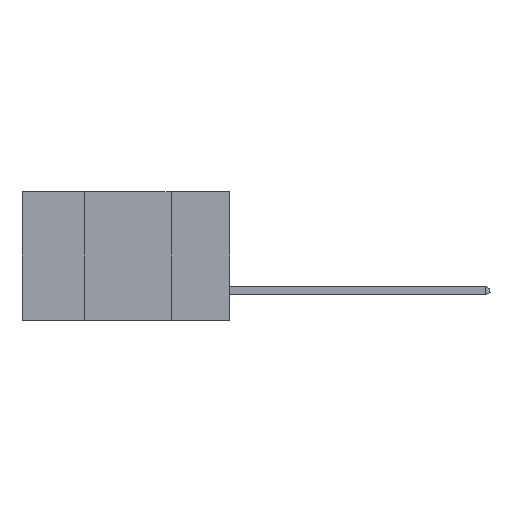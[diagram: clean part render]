
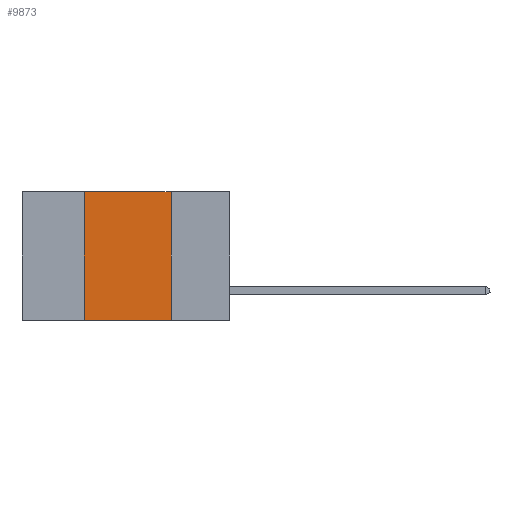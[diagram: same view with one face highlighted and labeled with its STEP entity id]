
A CAD part, left-side view. The second image highlights one B-rep face of the part: STEP entity #9873.
In plain terms, the highlighted planar face has unit normal (-1, 0, 0).
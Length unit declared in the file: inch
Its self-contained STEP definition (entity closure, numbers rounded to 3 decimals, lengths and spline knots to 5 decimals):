
#58 = CARTESIAN_POINT ( 'NONE',  ( 0., 0.17, 0. ) ) ;
#484 = CARTESIAN_POINT ( 'NONE',  ( 0., 0.17, 0. ) ) ;
#572 = DIRECTION ( 'NONE',  ( 0., 0., 1. ) ) ;
#2929 = VECTOR ( 'NONE', #15960, 39.37008 ) ;
#3571 = EDGE_CURVE ( 'NONE', #3934, #4231, #15487, .T. ) ;
#3934 = VERTEX_POINT ( 'NONE', #58 ) ;
#4231 = VERTEX_POINT ( 'NONE', #26623 ) ;
#5551 = ORIENTED_EDGE ( 'NONE', *, *, #24492, .F. ) ;
#6650 = VERTEX_POINT ( 'NONE', #12173 ) ;
#8415 = CARTESIAN_POINT ( 'NONE',  ( 0., 0.6, 0. ) ) ;
#8719 = CARTESIAN_POINT ( 'NONE',  ( 0., 0.42, -0.37 ) ) ;
#9023 = FACE_OUTER_BOUND ( 'NONE', #14346, .T. ) ;
#9120 = EDGE_CURVE ( 'NONE', #6650, #3934, #11376, .T. ) ;
#9525 = DIRECTION ( 'NONE',  ( 0., 0., -1. ) ) ;
#9628 = DIRECTION ( 'NONE',  ( 1., 0., 0. ) ) ;
#9873 = ADVANCED_FACE ( 'NONE', ( #9023 ), #26994, .F. ) ;
#11376 = LINE ( 'NONE', #8415, #2929 ) ;
#11632 = VECTOR ( 'NONE', #15706, 39.37008 ) ;
#11852 = EDGE_CURVE ( 'NONE', #23178, #4231, #27084, .T. ) ;
#12173 = CARTESIAN_POINT ( 'NONE',  ( 0., 0.42, 0. ) ) ;
#12731 = DIRECTION ( 'NONE',  ( 0., 0., -1. ) ) ;
#14346 = EDGE_LOOP ( 'NONE', ( #16572, #26202, #5551, #31586 ) ) ;
#14710 = VECTOR ( 'NONE', #12731, 39.37008 ) ;
#15487 = LINE ( 'NONE', #484, #14710 ) ;
#15499 = VECTOR ( 'NONE', #572, 39.37008 ) ;
#15706 = DIRECTION ( 'NONE',  ( 0., -1., 0. ) ) ;
#15960 = DIRECTION ( 'NONE',  ( 0., -1., 0. ) ) ;
#16572 = ORIENTED_EDGE ( 'NONE', *, *, #3571, .F. ) ;
#20145 = LINE ( 'NONE', #29883, #15499 ) ;
#23178 = VERTEX_POINT ( 'NONE', #8719 ) ;
#23602 = AXIS2_PLACEMENT_3D ( 'NONE', #24301, #9628, #9525 ) ;
#24301 = CARTESIAN_POINT ( 'NONE',  ( 0., 0.6, 0. ) ) ;
#24492 = EDGE_CURVE ( 'NONE', #23178, #6650, #20145, .T. ) ;
#26202 = ORIENTED_EDGE ( 'NONE', *, *, #9120, .F. ) ;
#26623 = CARTESIAN_POINT ( 'NONE',  ( 0., 0.17, -0.37 ) ) ;
#26994 = PLANE ( 'NONE',  #23602 ) ;
#27084 = LINE ( 'NONE', #30513, #11632 ) ;
#29883 = CARTESIAN_POINT ( 'NONE',  ( 0., 0.42, 0. ) ) ;
#30513 = CARTESIAN_POINT ( 'NONE',  ( 0., 0.6, -0.37 ) ) ;
#31586 = ORIENTED_EDGE ( 'NONE', *, *, #11852, .T. ) ;
